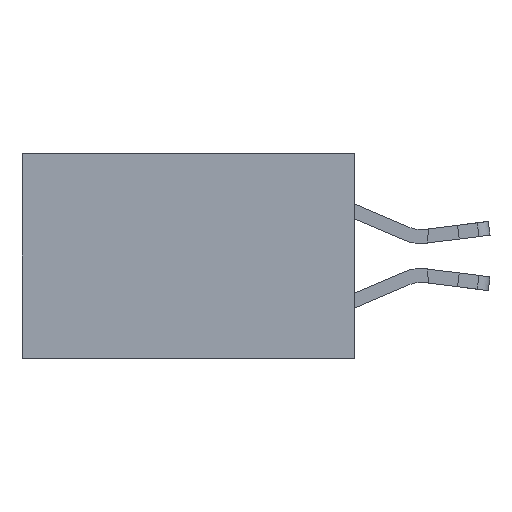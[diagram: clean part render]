
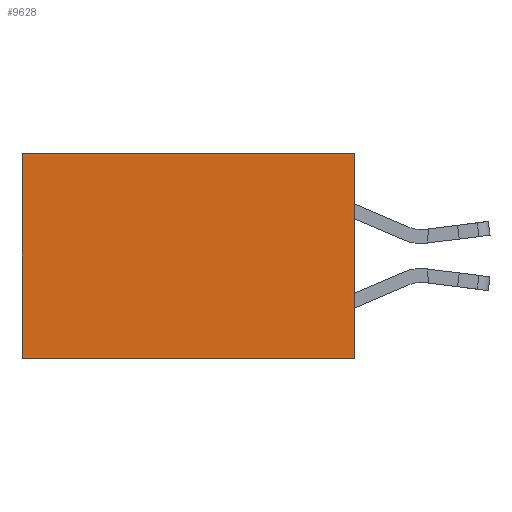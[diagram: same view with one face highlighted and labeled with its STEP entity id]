
A CAD part, left-side view. The second image highlights one B-rep face of the part: STEP entity #9628.
In plain terms, the highlighted planar face has unit normal (-1, 0, 0).
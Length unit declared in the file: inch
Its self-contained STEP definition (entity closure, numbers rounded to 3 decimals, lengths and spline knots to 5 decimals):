
#29 = ORIENTED_EDGE ( 'NONE', *, *, #221, .T. ) ;
#221 = EDGE_CURVE ( 'NONE', #3517, #5918, #5476, .T. ) ;
#254 = VERTEX_POINT ( 'NONE', #13705 ) ;
#485 = AXIS2_PLACEMENT_3D ( 'NONE', #8356, #2878, #2835 ) ;
#648 = PLANE ( 'NONE',  #485 ) ;
#710 = VECTOR ( 'NONE', #10082, 39.37008 ) ;
#1136 = VERTEX_POINT ( 'NONE', #4524 ) ;
#2497 = FACE_OUTER_BOUND ( 'NONE', #4096, .T. ) ;
#2668 = VECTOR ( 'NONE', #12296, 39.37008 ) ;
#2835 = DIRECTION ( 'NONE',  ( 0., 0., -1. ) ) ;
#2878 = DIRECTION ( 'NONE',  ( 1., 0., 0. ) ) ;
#2989 = CARTESIAN_POINT ( 'NONE',  ( 0.298, 0.6, 0. ) ) ;
#3357 = EDGE_CURVE ( 'NONE', #1136, #3517, #12830, .T. ) ;
#3517 = VERTEX_POINT ( 'NONE', #2989 ) ;
#4096 = EDGE_LOOP ( 'NONE', ( #29, #13378, #7653, #10752 ) ) ;
#4257 = VECTOR ( 'NONE', #10535, 39.37008 ) ;
#4524 = CARTESIAN_POINT ( 'NONE',  ( 0.298, 0., 0. ) ) ;
#4550 = CARTESIAN_POINT ( 'NONE',  ( 0.298, 0., 0. ) ) ;
#5245 = EDGE_CURVE ( 'NONE', #1136, #254, #11475, .T. ) ;
#5476 = LINE ( 'NONE', #12292, #2668 ) ;
#5918 = VERTEX_POINT ( 'NONE', #10354 ) ;
#6055 = EDGE_CURVE ( 'NONE', #254, #5918, #9039, .T. ) ;
#6508 = CARTESIAN_POINT ( 'NONE',  ( 0.298, 0., 0. ) ) ;
#7068 = VECTOR ( 'NONE', #9702, 39.37008 ) ;
#7653 = ORIENTED_EDGE ( 'NONE', *, *, #5245, .F. ) ;
#8356 = CARTESIAN_POINT ( 'NONE',  ( 0.298, 0., 0. ) ) ;
#9039 = LINE ( 'NONE', #10596, #710 ) ;
#9628 = ADVANCED_FACE ( 'NONE', ( #2497 ), #648, .F. ) ;
#9702 = DIRECTION ( 'NONE',  ( 0., 0., -1. ) ) ;
#10082 = DIRECTION ( 'NONE',  ( 0., 1., 0. ) ) ;
#10354 = CARTESIAN_POINT ( 'NONE',  ( 0.298, 0.6, -0.37 ) ) ;
#10535 = DIRECTION ( 'NONE',  ( 0., 1., 0. ) ) ;
#10596 = CARTESIAN_POINT ( 'NONE',  ( 0.298, 0., -0.37 ) ) ;
#10752 = ORIENTED_EDGE ( 'NONE', *, *, #3357, .T. ) ;
#11475 = LINE ( 'NONE', #6508, #7068 ) ;
#12292 = CARTESIAN_POINT ( 'NONE',  ( 0.298, 0.6, 0. ) ) ;
#12296 = DIRECTION ( 'NONE',  ( 0., 0., -1. ) ) ;
#12830 = LINE ( 'NONE', #4550, #4257 ) ;
#13378 = ORIENTED_EDGE ( 'NONE', *, *, #6055, .F. ) ;
#13705 = CARTESIAN_POINT ( 'NONE',  ( 0.298, 0., -0.37 ) ) ;
